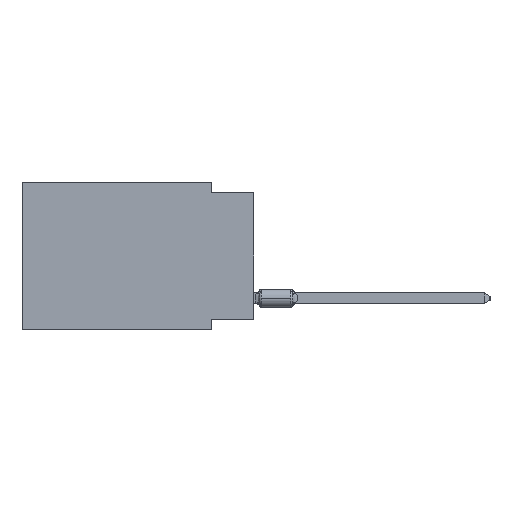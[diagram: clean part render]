
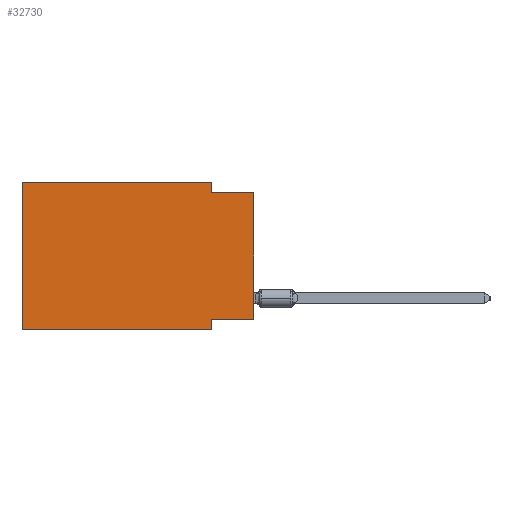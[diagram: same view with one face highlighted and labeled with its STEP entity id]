
A CAD part, left-side view. The second image highlights one B-rep face of the part: STEP entity #32730.
In plain terms, the highlighted planar face has unit normal (-1, 0, 0).
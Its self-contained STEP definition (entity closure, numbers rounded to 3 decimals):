
#901 = ORIENTED_EDGE ( 'NONE', *, *, #57491, .F. ) ;
#1966 = DIRECTION ( 'NONE',  ( 0., 0., 1. ) ) ;
#2152 = ORIENTED_EDGE ( 'NONE', *, *, #52603, .F. ) ;
#2162 = VECTOR ( 'NONE', #5692, 1000. ) ;
#2554 = CARTESIAN_POINT ( 'NONE',  ( 0., 2.54, 0. ) ) ;
#5692 = DIRECTION ( 'NONE',  ( 0., 0., 1. ) ) ;
#6720 = LINE ( 'NONE', #36347, #18697 ) ;
#7929 = DIRECTION ( 'NONE',  ( 0., 1., 0. ) ) ;
#8575 = PLANE ( 'NONE',  #57006 ) ;
#9096 = VERTEX_POINT ( 'NONE', #17098 ) ;
#9209 = ORIENTED_EDGE ( 'NONE', *, *, #15683, .F. ) ;
#9894 = EDGE_LOOP ( 'NONE', ( #13615, #901, #48549, #29534, #2152, #23948, #46553, #9209 ) ) ;
#10376 = LINE ( 'NONE', #48480, #2162 ) ;
#10555 = VECTOR ( 'NONE', #32243, 1000. ) ;
#10993 = CARTESIAN_POINT ( 'NONE',  ( 0., 0., -8.255 ) ) ;
#12664 = VERTEX_POINT ( 'NONE', #29846 ) ;
#13230 = LINE ( 'NONE', #56606, #10555 ) ;
#13464 = EDGE_CURVE ( 'NONE', #39950, #12664, #13883, .T. ) ;
#13615 = ORIENTED_EDGE ( 'NONE', *, *, #31355, .T. ) ;
#13883 = LINE ( 'NONE', #14810, #46372 ) ;
#14810 = CARTESIAN_POINT ( 'NONE',  ( 0., 13.97, -8.89 ) ) ;
#15683 = EDGE_CURVE ( 'NONE', #24512, #40755, #6720, .T. ) ;
#15898 = VECTOR ( 'NONE', #39559, 1000. ) ;
#16058 = LINE ( 'NONE', #35069, #29452 ) ;
#17098 = CARTESIAN_POINT ( 'NONE',  ( 0., 13.97, 0. ) ) ;
#18288 = DIRECTION ( 'NONE',  ( 1., 0., 0. ) ) ;
#18697 = VECTOR ( 'NONE', #7929, 1000. ) ;
#18887 = DIRECTION ( 'NONE',  ( 0., -1., 0. ) ) ;
#22964 = VERTEX_POINT ( 'NONE', #54467 ) ;
#23948 = ORIENTED_EDGE ( 'NONE', *, *, #13464, .T. ) ;
#24512 = VERTEX_POINT ( 'NONE', #10993 ) ;
#25480 = VERTEX_POINT ( 'NONE', #59535 ) ;
#26293 = LINE ( 'NONE', #2554, #35585 ) ;
#29030 = CARTESIAN_POINT ( 'NONE',  ( 0., 13.97, -8.89 ) ) ;
#29452 = VECTOR ( 'NONE', #1966, 1000. ) ;
#29534 = ORIENTED_EDGE ( 'NONE', *, *, #48401, .F. ) ;
#29846 = CARTESIAN_POINT ( 'NONE',  ( 0., 2.54, -8.89 ) ) ;
#31355 = EDGE_CURVE ( 'NONE', #24512, #40511, #10376, .T. ) ;
#32243 = DIRECTION ( 'NONE',  ( 0., -1., 0. ) ) ;
#32730 = ADVANCED_FACE ( 'NONE', ( #40430 ), #8575, .F. ) ;
#35069 = CARTESIAN_POINT ( 'NONE',  ( 0., 13.97, 0. ) ) ;
#35585 = VECTOR ( 'NONE', #45030, 1000. ) ;
#36347 = CARTESIAN_POINT ( 'NONE',  ( 0., 0., -8.255 ) ) ;
#37283 = DIRECTION ( 'NONE',  ( 0., 0., -1. ) ) ;
#39559 = DIRECTION ( 'NONE',  ( 0., -1., 0. ) ) ;
#39950 = VERTEX_POINT ( 'NONE', #29030 ) ;
#40430 = FACE_OUTER_BOUND ( 'NONE', #9894, .T. ) ;
#40511 = VERTEX_POINT ( 'NONE', #58802 ) ;
#40755 = VERTEX_POINT ( 'NONE', #44094 ) ;
#44094 = CARTESIAN_POINT ( 'NONE',  ( 0., 2.54, -8.255 ) ) ;
#44960 = EDGE_CURVE ( 'NONE', #22964, #25480, #26293, .T. ) ;
#45030 = DIRECTION ( 'NONE',  ( 0., 0., -1. ) ) ;
#45639 = LINE ( 'NONE', #49126, #60539 ) ;
#46372 = VECTOR ( 'NONE', #18887, 1000. ) ;
#46553 = ORIENTED_EDGE ( 'NONE', *, *, #59574, .F. ) ;
#48401 = EDGE_CURVE ( 'NONE', #9096, #22964, #13230, .T. ) ;
#48480 = CARTESIAN_POINT ( 'NONE',  ( 0., 0., 0. ) ) ;
#48549 = ORIENTED_EDGE ( 'NONE', *, *, #44960, .F. ) ;
#49126 = CARTESIAN_POINT ( 'NONE',  ( 0., 2.54, -8.89 ) ) ;
#52002 = CARTESIAN_POINT ( 'NONE',  ( 0., 13.97, 0. ) ) ;
#52603 = EDGE_CURVE ( 'NONE', #39950, #9096, #16058, .T. ) ;
#53950 = CARTESIAN_POINT ( 'NONE',  ( 0., 0., -0.635 ) ) ;
#54409 = DIRECTION ( 'NONE',  ( 0., 0., -1. ) ) ;
#54467 = CARTESIAN_POINT ( 'NONE',  ( 0., 2.54, 0. ) ) ;
#56606 = CARTESIAN_POINT ( 'NONE',  ( 0., 13.97, 0. ) ) ;
#57006 = AXIS2_PLACEMENT_3D ( 'NONE', #52002, #18288, #37283 ) ;
#57491 = EDGE_CURVE ( 'NONE', #25480, #40511, #58011, .T. ) ;
#58011 = LINE ( 'NONE', #53950, #15898 ) ;
#58802 = CARTESIAN_POINT ( 'NONE',  ( 0., 0., -0.635 ) ) ;
#59535 = CARTESIAN_POINT ( 'NONE',  ( 0., 2.54, -0.635 ) ) ;
#59574 = EDGE_CURVE ( 'NONE', #40755, #12664, #45639, .T. ) ;
#60539 = VECTOR ( 'NONE', #54409, 1000. ) ;
